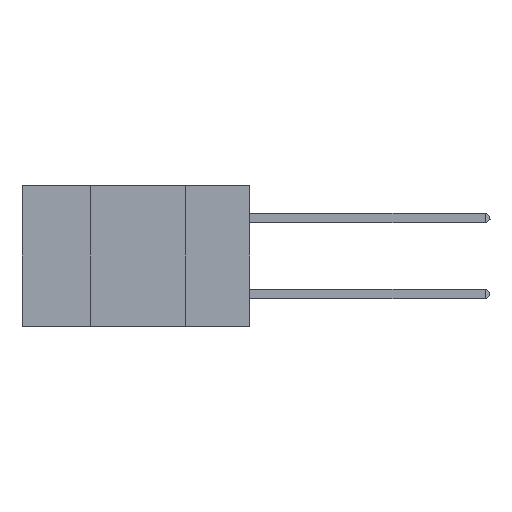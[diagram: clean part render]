
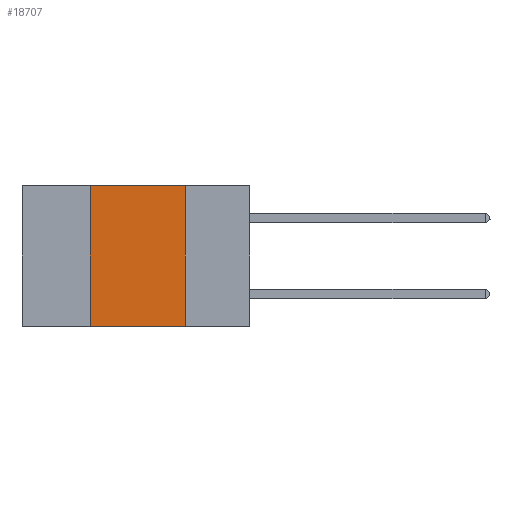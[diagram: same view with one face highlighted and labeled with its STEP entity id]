
A CAD part, left-side view. The second image highlights one B-rep face of the part: STEP entity #18707.
In plain terms, the highlighted planar face has unit normal (-1, 0, 0).
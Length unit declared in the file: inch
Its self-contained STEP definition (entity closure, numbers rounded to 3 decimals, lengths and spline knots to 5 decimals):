
#154 = EDGE_CURVE ( 'NONE', #13245, #2680, #10337, .T. ) ;
#214 = LINE ( 'NONE', #17867, #18794 ) ;
#618 = EDGE_CURVE ( 'NONE', #13245, #16744, #19162, .T. ) ;
#890 = CARTESIAN_POINT ( 'NONE',  ( 0., 0.17, 0. ) ) ;
#1385 = VECTOR ( 'NONE', #16359, 39.37008 ) ;
#2680 = VERTEX_POINT ( 'NONE', #3942 ) ;
#3942 = CARTESIAN_POINT ( 'NONE',  ( 0., 0.17, -0.37 ) ) ;
#4369 = ORIENTED_EDGE ( 'NONE', *, *, #10501, .F. ) ;
#4477 = CARTESIAN_POINT ( 'NONE',  ( 0., 0.42, 0. ) ) ;
#4701 = CARTESIAN_POINT ( 'NONE',  ( 0., 0.6, 0. ) ) ;
#5096 = ORIENTED_EDGE ( 'NONE', *, *, #17627, .F. ) ;
#5422 = VECTOR ( 'NONE', #5957, 39.37008 ) ;
#5793 = EDGE_LOOP ( 'NONE', ( #5096, #4369, #16094, #15620 ) ) ;
#5957 = DIRECTION ( 'NONE',  ( 0., -1., 0. ) ) ;
#6240 = CARTESIAN_POINT ( 'NONE',  ( 0., 0.6, -0.37 ) ) ;
#6963 = CARTESIAN_POINT ( 'NONE',  ( 0., 0.42, -0.37 ) ) ;
#7621 = FACE_OUTER_BOUND ( 'NONE', #5793, .T. ) ;
#7944 = VERTEX_POINT ( 'NONE', #14829 ) ;
#8376 = VECTOR ( 'NONE', #9559, 39.37008 ) ;
#8402 = AXIS2_PLACEMENT_3D ( 'NONE', #4701, #10833, #18043 ) ;
#9559 = DIRECTION ( 'NONE',  ( 0., 0., -1. ) ) ;
#10337 = LINE ( 'NONE', #6240, #5422 ) ;
#10462 = DIRECTION ( 'NONE',  ( 0., -1., 0. ) ) ;
#10501 = EDGE_CURVE ( 'NONE', #16744, #7944, #214, .T. ) ;
#10833 = DIRECTION ( 'NONE',  ( 1., 0., 0. ) ) ;
#12005 = PLANE ( 'NONE',  #8402 ) ;
#13245 = VERTEX_POINT ( 'NONE', #6963 ) ;
#14829 = CARTESIAN_POINT ( 'NONE',  ( 0., 0.17, 0. ) ) ;
#15314 = LINE ( 'NONE', #890, #8376 ) ;
#15620 = ORIENTED_EDGE ( 'NONE', *, *, #154, .T. ) ;
#16094 = ORIENTED_EDGE ( 'NONE', *, *, #618, .F. ) ;
#16359 = DIRECTION ( 'NONE',  ( 0., 0., 1. ) ) ;
#16744 = VERTEX_POINT ( 'NONE', #17212 ) ;
#17212 = CARTESIAN_POINT ( 'NONE',  ( 0., 0.42, 0. ) ) ;
#17627 = EDGE_CURVE ( 'NONE', #7944, #2680, #15314, .T. ) ;
#17867 = CARTESIAN_POINT ( 'NONE',  ( 0., 0.6, 0. ) ) ;
#18043 = DIRECTION ( 'NONE',  ( 0., 0., -1. ) ) ;
#18707 = ADVANCED_FACE ( 'NONE', ( #7621 ), #12005, .F. ) ;
#18794 = VECTOR ( 'NONE', #10462, 39.37008 ) ;
#19162 = LINE ( 'NONE', #4477, #1385 ) ;
